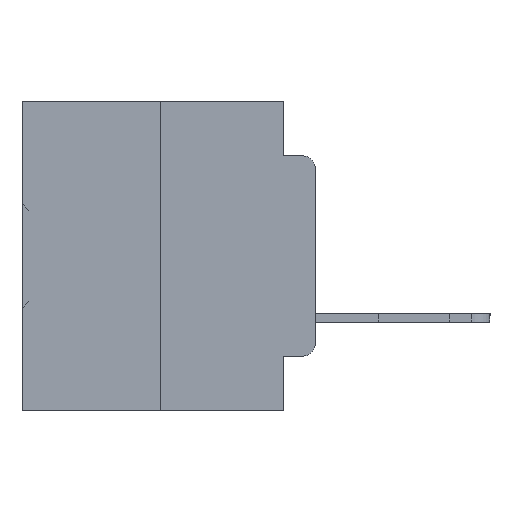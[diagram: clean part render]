
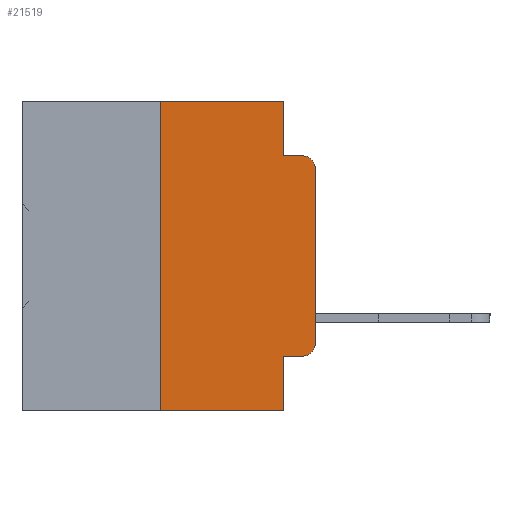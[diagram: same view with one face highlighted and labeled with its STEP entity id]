
A CAD part, left-side view. The second image highlights one B-rep face of the part: STEP entity #21519.
In plain terms, the highlighted planar face has unit normal (-1, 0, 0).
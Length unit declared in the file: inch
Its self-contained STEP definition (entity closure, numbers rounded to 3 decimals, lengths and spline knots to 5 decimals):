
#249 = CARTESIAN_POINT ( 'NONE',  ( 0., 0.051, -0.5 ) ) ;
#1647 = CARTESIAN_POINT ( 'NONE',  ( 0., 0.051, -0.0885 ) ) ;
#2897 = CARTESIAN_POINT ( 'NONE',  ( 0., 0.051, -0.4115 ) ) ;
#3663 = CARTESIAN_POINT ( 'NONE',  ( 0., 0.02, -0.3915 ) ) ;
#4188 = EDGE_LOOP ( 'NONE', ( #16153, #29943, #32373, #19204, #29934, #13752, #4462, #14462, #8747, #27546 ) ) ;
#4462 = ORIENTED_EDGE ( 'NONE', *, *, #20142, .T. ) ;
#5113 = LINE ( 'NONE', #1647, #26323 ) ;
#5437 = CARTESIAN_POINT ( 'NONE',  ( 0., 0.051, 0. ) ) ;
#5832 = VERTEX_POINT ( 'NONE', #13272 ) ;
#6083 = VERTEX_POINT ( 'NONE', #11399 ) ;
#6361 = VERTEX_POINT ( 'NONE', #2897 ) ;
#6593 = DIRECTION ( 'NONE',  ( 0., 0., -1. ) ) ;
#6735 = LINE ( 'NONE', #12311, #29645 ) ;
#7302 = VECTOR ( 'NONE', #14419, 39.37008 ) ;
#8220 = LINE ( 'NONE', #34415, #7302 ) ;
#8241 = LINE ( 'NONE', #32332, #36875 ) ;
#8747 = ORIENTED_EDGE ( 'NONE', *, *, #23673, .T. ) ;
#9420 = VERTEX_POINT ( 'NONE', #15970 ) ;
#9570 = DIRECTION ( 'NONE',  ( 0., -1., 0. ) ) ;
#9733 = CARTESIAN_POINT ( 'NONE',  ( 0., 0.25, 0. ) ) ;
#10627 = LINE ( 'NONE', #5437, #25007 ) ;
#11035 = CARTESIAN_POINT ( 'NONE',  ( 0., 0.473, 0. ) ) ;
#11169 = EDGE_CURVE ( 'NONE', #29223, #24478, #15031, .T. ) ;
#11399 = CARTESIAN_POINT ( 'NONE',  ( 0., 0.051, -0.0885 ) ) ;
#11662 = EDGE_CURVE ( 'NONE', #34481, #6083, #8220, .T. ) ;
#12311 = CARTESIAN_POINT ( 'NONE',  ( 0., 0.051, -0.4115 ) ) ;
#12580 = AXIS2_PLACEMENT_3D ( 'NONE', #11035, #36786, #19719 ) ;
#12891 = AXIS2_PLACEMENT_3D ( 'NONE', #3663, #23875, #6593 ) ;
#13272 = CARTESIAN_POINT ( 'NONE',  ( 0., 0., -0.1085 ) ) ;
#13499 = CARTESIAN_POINT ( 'NONE',  ( 0., 0., -0.3915 ) ) ;
#13752 = ORIENTED_EDGE ( 'NONE', *, *, #27716, .F. ) ;
#14128 = VERTEX_POINT ( 'NONE', #9733 ) ;
#14419 = DIRECTION ( 'NONE',  ( 0., 0., -1. ) ) ;
#14462 = ORIENTED_EDGE ( 'NONE', *, *, #37214, .F. ) ;
#14727 = LINE ( 'NONE', #21384, #29054 ) ;
#15031 = CIRCLE ( 'NONE', #12891, 0.02 ) ;
#15127 = CARTESIAN_POINT ( 'NONE',  ( 0., 0.25, -0.5 ) ) ;
#15419 = VERTEX_POINT ( 'NONE', #15127 ) ;
#15970 = CARTESIAN_POINT ( 'NONE',  ( 0., 0.02, -0.0885 ) ) ;
#16153 = ORIENTED_EDGE ( 'NONE', *, *, #35613, .T. ) ;
#16906 = CARTESIAN_POINT ( 'NONE',  ( 0., 0.02, -0.1085 ) ) ;
#16988 = EDGE_CURVE ( 'NONE', #5832, #9420, #26707, .T. ) ;
#17301 = CARTESIAN_POINT ( 'NONE',  ( 0., 0.02, -0.4115 ) ) ;
#17765 = FACE_OUTER_BOUND ( 'NONE', #4188, .T. ) ;
#17974 = EDGE_CURVE ( 'NONE', #14128, #34481, #8241, .T. ) ;
#19204 = ORIENTED_EDGE ( 'NONE', *, *, #11662, .F. ) ;
#19719 = DIRECTION ( 'NONE',  ( 0., 0., -1. ) ) ;
#19777 = DIRECTION ( 'NONE',  ( 0., 0., -1. ) ) ;
#20142 = EDGE_CURVE ( 'NONE', #15419, #25416, #30920, .T. ) ;
#20657 = VECTOR ( 'NONE', #32542, 39.37008 ) ;
#21384 = CARTESIAN_POINT ( 'NONE',  ( 0., 0.25, 0. ) ) ;
#21519 = ADVANCED_FACE ( 'NONE', ( #17765 ), #25371, .F. ) ;
#22451 = VECTOR ( 'NONE', #28834, 39.37008 ) ;
#23673 = EDGE_CURVE ( 'NONE', #6361, #29223, #6735, .T. ) ;
#23875 = DIRECTION ( 'NONE',  ( -1., 0., 0. ) ) ;
#24283 = DIRECTION ( 'NONE',  ( 0., 0., 1. ) ) ;
#24478 = VERTEX_POINT ( 'NONE', #13499 ) ;
#24736 = DIRECTION ( 'NONE',  ( 0., -1., 0. ) ) ;
#25007 = VECTOR ( 'NONE', #28465, 39.37008 ) ;
#25371 = PLANE ( 'NONE',  #12580 ) ;
#25416 = VERTEX_POINT ( 'NONE', #249 ) ;
#25989 = CARTESIAN_POINT ( 'NONE',  ( 0., 0.473, -0.5 ) ) ;
#26323 = VECTOR ( 'NONE', #24736, 39.37008 ) ;
#26597 = EDGE_CURVE ( 'NONE', #6083, #9420, #5113, .T. ) ;
#26707 = CIRCLE ( 'NONE', #33178, 0.02 ) ;
#27546 = ORIENTED_EDGE ( 'NONE', *, *, #11169, .T. ) ;
#27716 = EDGE_CURVE ( 'NONE', #15419, #14128, #14727, .T. ) ;
#28465 = DIRECTION ( 'NONE',  ( 0., 0., -1. ) ) ;
#28538 = CARTESIAN_POINT ( 'NONE',  ( 0., 0.051, 0. ) ) ;
#28834 = DIRECTION ( 'NONE',  ( 0., -1., 0. ) ) ;
#29054 = VECTOR ( 'NONE', #24283, 39.37008 ) ;
#29223 = VERTEX_POINT ( 'NONE', #17301 ) ;
#29456 = DIRECTION ( 'NONE',  ( 0., -1., 0. ) ) ;
#29645 = VECTOR ( 'NONE', #29456, 39.37008 ) ;
#29672 = CARTESIAN_POINT ( 'NONE',  ( 0., 0., 0. ) ) ;
#29934 = ORIENTED_EDGE ( 'NONE', *, *, #17974, .F. ) ;
#29943 = ORIENTED_EDGE ( 'NONE', *, *, #16988, .T. ) ;
#30920 = LINE ( 'NONE', #25989, #22451 ) ;
#32332 = CARTESIAN_POINT ( 'NONE',  ( 0., 0.473, 0. ) ) ;
#32373 = ORIENTED_EDGE ( 'NONE', *, *, #26597, .F. ) ;
#32542 = DIRECTION ( 'NONE',  ( 0., 0., 1. ) ) ;
#33178 = AXIS2_PLACEMENT_3D ( 'NONE', #16906, #36836, #19777 ) ;
#34415 = CARTESIAN_POINT ( 'NONE',  ( 0., 0.051, 0. ) ) ;
#34481 = VERTEX_POINT ( 'NONE', #28538 ) ;
#35613 = EDGE_CURVE ( 'NONE', #24478, #5832, #35805, .T. ) ;
#35805 = LINE ( 'NONE', #29672, #20657 ) ;
#36786 = DIRECTION ( 'NONE',  ( 1., 0., 0. ) ) ;
#36836 = DIRECTION ( 'NONE',  ( -1., 0., 0. ) ) ;
#36875 = VECTOR ( 'NONE', #9570, 39.37008 ) ;
#37214 = EDGE_CURVE ( 'NONE', #6361, #25416, #10627, .T. ) ;
